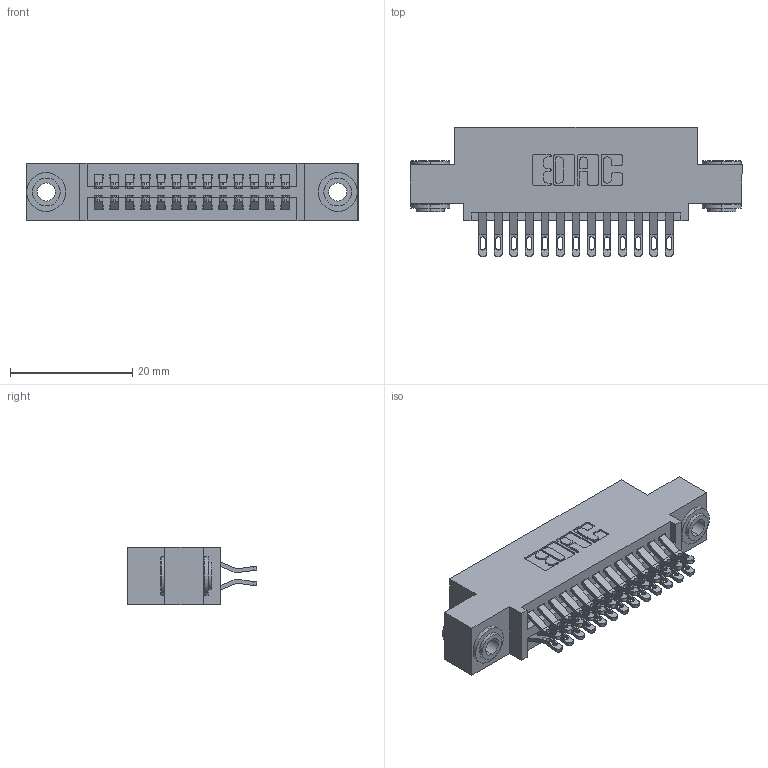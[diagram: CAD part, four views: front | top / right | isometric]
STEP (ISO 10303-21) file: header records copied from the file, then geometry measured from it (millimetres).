
FILE_DESCRIPTION (( 'STEP AP203' ), '1' );
FILE_NAME ('395-026-555-503.STEP', '2018-11-10T00:53:17', ( '' ), ( '' ), 'SwSTEP 2.0', 'SolidWorks 2016', '' );
FILE_SCHEMA (( 'CONFIG_CONTROL_DESIGN' ));
Length unit declared in the file: inch
Products named in the file (4): 345-292-001_555 Tail; 345-250-002_345-250-002-102; 345 Part_0.110 Offset - 0.156 Dia-TH; 395-026-555-503
Assembly tree (29 placements, depth 2):
  395-026-555-503
    345 Part_0.110 Offset - 0.156 Dia-TH
    345-292-001_555 Tail  x26
    345-250-002_345-250-002-102  x2
Bounding box: 54.23 x 21.13 x 9.4 mm (x, y, z)
Volume: 5020.1 mm3; surface area: 7418.9 mm2
Topology: 29 solids, 29 shells, 1624 faces, 5031 edges, 3350 vertices
Faces by surface type: plane 900, cylinder 716, cone 8
Entity records: 15212 total; most frequent: CARTESIAN_POINT 2589, ORIENTED_EDGE 2486, DIRECTION 2317, EDGE_CURVE 1243, VECTOR 1015, LINE 1015, VERTEX_POINT 826, AXIS2_PLACEMENT_3D 651
